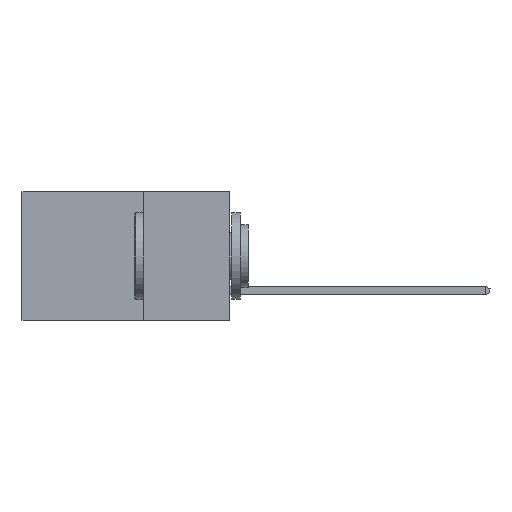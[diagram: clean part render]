
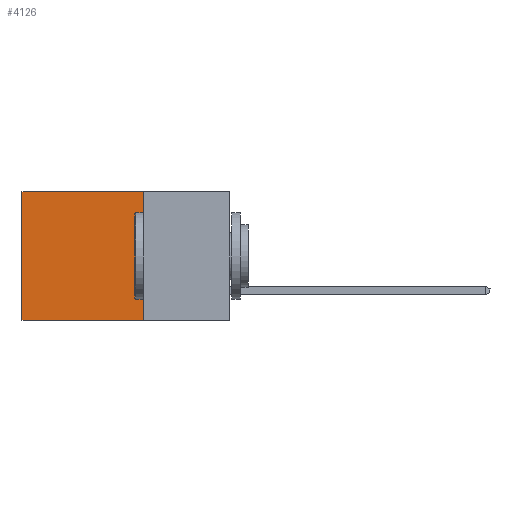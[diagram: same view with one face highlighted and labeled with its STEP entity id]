
A CAD part, left-side view. The second image highlights one B-rep face of the part: STEP entity #4126.
In plain terms, the highlighted planar face has unit normal (-1, 0, 0).
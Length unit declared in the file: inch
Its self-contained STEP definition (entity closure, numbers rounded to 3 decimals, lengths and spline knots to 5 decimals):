
#22 = DIRECTION ( 'NONE',  ( 0., 0., -1. ) ) ;
#400 = AXIS2_PLACEMENT_3D ( 'NONE', #7827, #7879, #8671 ) ;
#473 = VERTEX_POINT ( 'NONE', #5962 ) ;
#1233 = LINE ( 'NONE', #7710, #9610 ) ;
#1409 = VECTOR ( 'NONE', #5891, 39.37008 ) ;
#2531 = EDGE_CURVE ( 'NONE', #8719, #4395, #7528, .T. ) ;
#2841 = EDGE_LOOP ( 'NONE', ( #6812, #3882, #4572, #10257 ) ) ;
#3689 = CARTESIAN_POINT ( 'NONE',  ( 0.2615, 0.25, -0.37 ) ) ;
#3882 = ORIENTED_EDGE ( 'NONE', *, *, #2531, .F. ) ;
#4126 = ADVANCED_FACE ( 'NONE', ( #9370 ), #8722, .F. ) ;
#4367 = DIRECTION ( 'NONE',  ( 0., 0., -1. ) ) ;
#4395 = VERTEX_POINT ( 'NONE', #6830 ) ;
#4515 = CARTESIAN_POINT ( 'NONE',  ( 0.2615, 0.25, 0. ) ) ;
#4572 = ORIENTED_EDGE ( 'NONE', *, *, #10329, .F. ) ;
#5064 = EDGE_CURVE ( 'NONE', #473, #4395, #5843, .T. ) ;
#5843 = LINE ( 'NONE', #6749, #6673 ) ;
#5891 = DIRECTION ( 'NONE',  ( 0., 1., 0. ) ) ;
#5962 = CARTESIAN_POINT ( 'NONE',  ( 0.2615, 0.6, 0. ) ) ;
#5992 = CARTESIAN_POINT ( 'NONE',  ( 0.2615, 0.25, -0.37 ) ) ;
#6673 = VECTOR ( 'NONE', #4367, 39.37008 ) ;
#6749 = CARTESIAN_POINT ( 'NONE',  ( 0.2615, 0.6, -0.37 ) ) ;
#6801 = DIRECTION ( 'NONE',  ( 0., 1., 0. ) ) ;
#6812 = ORIENTED_EDGE ( 'NONE', *, *, #5064, .T. ) ;
#6830 = CARTESIAN_POINT ( 'NONE',  ( 0.2615, 0.6, -0.37 ) ) ;
#7528 = LINE ( 'NONE', #5992, #1409 ) ;
#7710 = CARTESIAN_POINT ( 'NONE',  ( 0.2615, 0.25, 0. ) ) ;
#7827 = CARTESIAN_POINT ( 'NONE',  ( 0.2615, 0.25, -0.37 ) ) ;
#7879 = DIRECTION ( 'NONE',  ( 1., 0., 0. ) ) ;
#7958 = LINE ( 'NONE', #10385, #9790 ) ;
#8671 = DIRECTION ( 'NONE',  ( 0., 0., -1. ) ) ;
#8719 = VERTEX_POINT ( 'NONE', #3689 ) ;
#8722 = PLANE ( 'NONE',  #400 ) ;
#9167 = VERTEX_POINT ( 'NONE', #4515 ) ;
#9370 = FACE_OUTER_BOUND ( 'NONE', #2841, .T. ) ;
#9610 = VECTOR ( 'NONE', #6801, 39.37008 ) ;
#9790 = VECTOR ( 'NONE', #22, 39.37008 ) ;
#10163 = EDGE_CURVE ( 'NONE', #9167, #473, #1233, .T. ) ;
#10257 = ORIENTED_EDGE ( 'NONE', *, *, #10163, .T. ) ;
#10329 = EDGE_CURVE ( 'NONE', #9167, #8719, #7958, .T. ) ;
#10385 = CARTESIAN_POINT ( 'NONE',  ( 0.2615, 0.25, -0.37 ) ) ;
